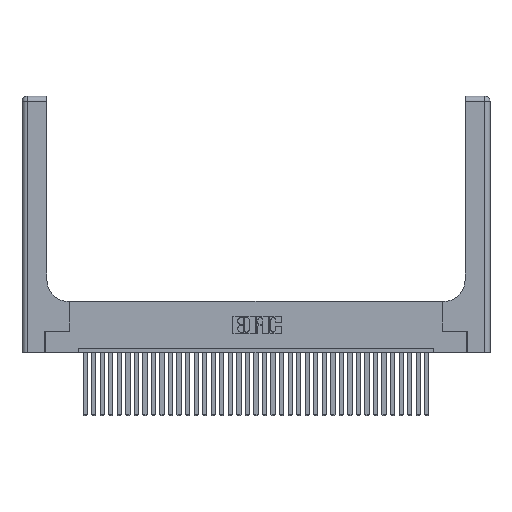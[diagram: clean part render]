
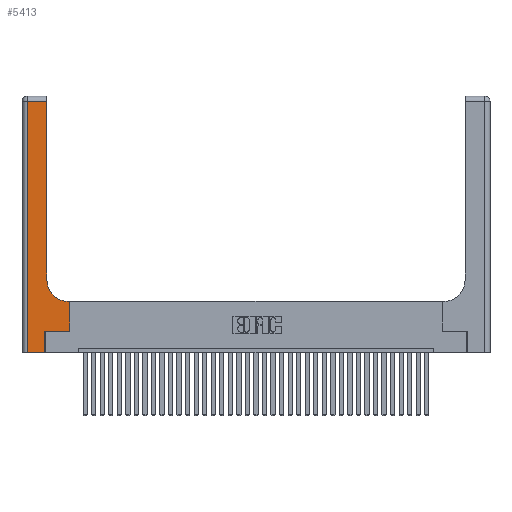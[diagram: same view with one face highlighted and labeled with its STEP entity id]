
A CAD part, top view. The second image highlights one B-rep face of the part: STEP entity #5413.
In plain terms, the highlighted planar face has unit normal (0, 0, 1).
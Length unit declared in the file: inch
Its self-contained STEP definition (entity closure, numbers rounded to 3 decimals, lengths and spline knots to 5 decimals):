
#316 = CARTESIAN_POINT ( 'NONE',  ( 0.5415, 0.6, 0.37 ) ) ;
#322 = EDGE_CURVE ( 'NONE', #30003, #24150, #33771, .T. ) ;
#1574 = ORIENTED_EDGE ( 'NONE', *, *, #10095, .T. ) ;
#2195 = FACE_OUTER_BOUND ( 'NONE', #25978, .T. ) ;
#2873 = CARTESIAN_POINT ( 'NONE',  ( 0.06, 0., 0.37 ) ) ;
#3423 = EDGE_CURVE ( 'NONE', #4569, #9155, #12766, .T. ) ;
#3576 = EDGE_CURVE ( 'NONE', #4717, #33915, #19740, .T. ) ;
#3896 = VECTOR ( 'NONE', #20232, 39.37008 ) ;
#4348 = VECTOR ( 'NONE', #22770, 39.37008 ) ;
#4410 = LINE ( 'NONE', #26072, #25748 ) ;
#4569 = VERTEX_POINT ( 'NONE', #4639 ) ;
#4639 = CARTESIAN_POINT ( 'NONE',  ( 0.2915, 2.94, 0.37 ) ) ;
#4690 = DIRECTION ( 'NONE',  ( 0., 0., -1. ) ) ;
#4717 = VERTEX_POINT ( 'NONE', #19355 ) ;
#4825 = VECTOR ( 'NONE', #27754, 39.37008 ) ;
#5316 = DIRECTION ( 'NONE',  ( 0., 0., -1. ) ) ;
#5397 = VECTOR ( 'NONE', #10776, 39.37008 ) ;
#5413 = ADVANCED_FACE ( 'NONE', ( #2195 ), #11764, .F. ) ;
#5712 = VERTEX_POINT ( 'NONE', #25761 ) ;
#5735 = CARTESIAN_POINT ( 'NONE',  ( 0.06, 3., 0.37 ) ) ;
#6294 = VECTOR ( 'NONE', #25008, 39.37008 ) ;
#8381 = EDGE_CURVE ( 'NONE', #29699, #5712, #9389, .T. ) ;
#9124 = ORIENTED_EDGE ( 'NONE', *, *, #322, .T. ) ;
#9155 = VERTEX_POINT ( 'NONE', #13601 ) ;
#9389 = CIRCLE ( 'NONE', #29551, 0.25 ) ;
#10095 = EDGE_CURVE ( 'NONE', #16027, #4717, #15143, .T. ) ;
#10102 = CARTESIAN_POINT ( 'NONE',  ( 0.269, 0., 0.37 ) ) ;
#10776 = DIRECTION ( 'NONE',  ( -1., 0., 0. ) ) ;
#10909 = LINE ( 'NONE', #5735, #4825 ) ;
#11159 = ORIENTED_EDGE ( 'NONE', *, *, #23553, .T. ) ;
#11312 = AXIS2_PLACEMENT_3D ( 'NONE', #14417, #5316, #19183 ) ;
#11567 = VECTOR ( 'NONE', #25345, 39.37008 ) ;
#11764 = PLANE ( 'NONE',  #11312 ) ;
#11883 = VECTOR ( 'NONE', #13937, 39.37008 ) ;
#12766 = LINE ( 'NONE', #21704, #5397 ) ;
#12945 = CARTESIAN_POINT ( 'NONE',  ( 0.5415, 0.85, 0.37 ) ) ;
#13027 = LINE ( 'NONE', #19140, #4348 ) ;
#13179 = DIRECTION ( 'NONE',  ( 1., 0., 0. ) ) ;
#13601 = CARTESIAN_POINT ( 'NONE',  ( 0.06, 2.94, 0.37 ) ) ;
#13937 = DIRECTION ( 'NONE',  ( 0., 1., 0. ) ) ;
#14233 = CARTESIAN_POINT ( 'NONE',  ( 0., 0., 0.37 ) ) ;
#14417 = CARTESIAN_POINT ( 'NONE',  ( 0., 3., 0.37 ) ) ;
#14522 = EDGE_CURVE ( 'NONE', #5712, #4569, #4410, .T. ) ;
#14657 = ORIENTED_EDGE ( 'NONE', *, *, #8381, .T. ) ;
#15143 = LINE ( 'NONE', #17558, #3896 ) ;
#16027 = VERTEX_POINT ( 'NONE', #34744 ) ;
#16529 = CARTESIAN_POINT ( 'NONE',  ( 0.5585, 0.25, 0.37 ) ) ;
#17558 = CARTESIAN_POINT ( 'NONE',  ( 0.269, 0.25, 0.37 ) ) ;
#19140 = CARTESIAN_POINT ( 'NONE',  ( 0.269, 0., 0.37 ) ) ;
#19183 = DIRECTION ( 'NONE',  ( -1., 0., 0. ) ) ;
#19355 = CARTESIAN_POINT ( 'NONE',  ( 0.5585, 0.25, 0.37 ) ) ;
#19740 = LINE ( 'NONE', #16529, #11883 ) ;
#20232 = DIRECTION ( 'NONE',  ( 1., 0., 0. ) ) ;
#21303 = ORIENTED_EDGE ( 'NONE', *, *, #3576, .T. ) ;
#21704 = CARTESIAN_POINT ( 'NONE',  ( 0., 2.94, 0.37 ) ) ;
#22770 = DIRECTION ( 'NONE',  ( 0., 1., 0. ) ) ;
#23553 = EDGE_CURVE ( 'NONE', #33915, #29699, #35410, .T. ) ;
#24150 = VERTEX_POINT ( 'NONE', #10102 ) ;
#24669 = CARTESIAN_POINT ( 'NONE',  ( 0.2915, 0.6, 0.37 ) ) ;
#25008 = DIRECTION ( 'NONE',  ( -1., 0., 0. ) ) ;
#25345 = DIRECTION ( 'NONE',  ( 1., 0., 0. ) ) ;
#25748 = VECTOR ( 'NONE', #34319, 39.37008 ) ;
#25761 = CARTESIAN_POINT ( 'NONE',  ( 0.2915, 0.85, 0.37 ) ) ;
#25978 = EDGE_LOOP ( 'NONE', ( #31496, #35128, #27656, #9124, #29626, #1574, #21303, #11159, #14657 ) ) ;
#26072 = CARTESIAN_POINT ( 'NONE',  ( 0.2915, 3., 0.37 ) ) ;
#27656 = ORIENTED_EDGE ( 'NONE', *, *, #35367, .T. ) ;
#27754 = DIRECTION ( 'NONE',  ( 0., -1., 0. ) ) ;
#29551 = AXIS2_PLACEMENT_3D ( 'NONE', #12945, #4690, #13179 ) ;
#29626 = ORIENTED_EDGE ( 'NONE', *, *, #29683, .T. ) ;
#29683 = EDGE_CURVE ( 'NONE', #24150, #16027, #13027, .T. ) ;
#29699 = VERTEX_POINT ( 'NONE', #316 ) ;
#30003 = VERTEX_POINT ( 'NONE', #2873 ) ;
#31496 = ORIENTED_EDGE ( 'NONE', *, *, #14522, .T. ) ;
#33771 = LINE ( 'NONE', #14233, #11567 ) ;
#33915 = VERTEX_POINT ( 'NONE', #34996 ) ;
#34319 = DIRECTION ( 'NONE',  ( 0., 1., 0. ) ) ;
#34744 = CARTESIAN_POINT ( 'NONE',  ( 0.269, 0.25, 0.37 ) ) ;
#34996 = CARTESIAN_POINT ( 'NONE',  ( 0.5585, 0.6, 0.37 ) ) ;
#35128 = ORIENTED_EDGE ( 'NONE', *, *, #3423, .T. ) ;
#35367 = EDGE_CURVE ( 'NONE', #9155, #30003, #10909, .T. ) ;
#35410 = LINE ( 'NONE', #24669, #6294 ) ;
